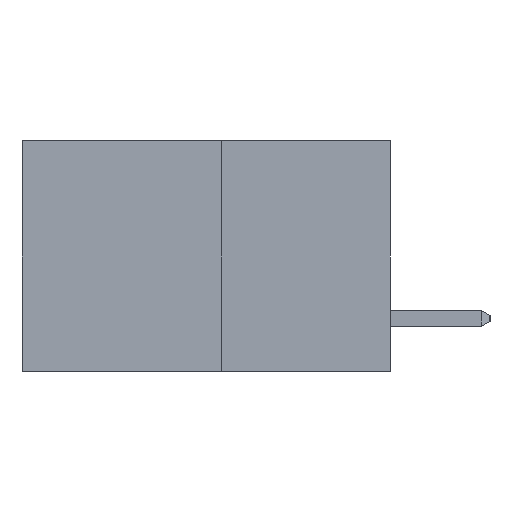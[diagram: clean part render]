
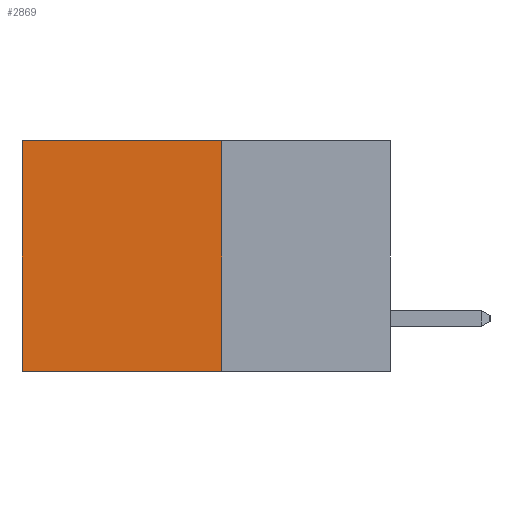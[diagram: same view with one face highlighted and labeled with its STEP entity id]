
A CAD part, left-side view. The second image highlights one B-rep face of the part: STEP entity #2869.
In plain terms, the highlighted planar face has unit normal (-1, 0, 0).
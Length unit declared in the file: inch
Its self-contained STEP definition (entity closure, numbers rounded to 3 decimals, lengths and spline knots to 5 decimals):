
#576 = LINE ( 'NONE', #3985, #7108 ) ;
#730 = DIRECTION ( 'NONE',  ( 0., 1., 0. ) ) ;
#1033 = CARTESIAN_POINT ( 'NONE',  ( 0.277, 0.59, -0.37 ) ) ;
#1286 = DIRECTION ( 'NONE',  ( 0., 0., -1. ) ) ;
#1570 = CARTESIAN_POINT ( 'NONE',  ( 0.277, 0.27, -0.37 ) ) ;
#1592 = LINE ( 'NONE', #6024, #7834 ) ;
#1625 = EDGE_LOOP ( 'NONE', ( #1772, #9178, #2655, #3775 ) ) ;
#1628 = VERTEX_POINT ( 'NONE', #6044 ) ;
#1671 = PLANE ( 'NONE',  #3320 ) ;
#1772 = ORIENTED_EDGE ( 'NONE', *, *, #9728, .T. ) ;
#1929 = VECTOR ( 'NONE', #8327, 39.37008 ) ;
#2655 = ORIENTED_EDGE ( 'NONE', *, *, #8608, .F. ) ;
#2869 = ADVANCED_FACE ( 'NONE', ( #3072 ), #1671, .F. ) ;
#3072 = FACE_OUTER_BOUND ( 'NONE', #1625, .T. ) ;
#3103 = CARTESIAN_POINT ( 'NONE',  ( 0.277, 0.27, 0. ) ) ;
#3320 = AXIS2_PLACEMENT_3D ( 'NONE', #1570, #6896, #9042 ) ;
#3775 = ORIENTED_EDGE ( 'NONE', *, *, #7392, .T. ) ;
#3849 = CARTESIAN_POINT ( 'NONE',  ( 0.277, 0.27, -0.37 ) ) ;
#3985 = CARTESIAN_POINT ( 'NONE',  ( 0.277, 0.27, 0. ) ) ;
#4096 = EDGE_CURVE ( 'NONE', #6271, #1628, #6357, .T. ) ;
#4168 = CARTESIAN_POINT ( 'NONE',  ( 0.277, 0.59, 0. ) ) ;
#4412 = VECTOR ( 'NONE', #9612, 39.37008 ) ;
#5174 = LINE ( 'NONE', #1033, #4412 ) ;
#5218 = VERTEX_POINT ( 'NONE', #4168 ) ;
#6024 = CARTESIAN_POINT ( 'NONE',  ( 0.277, 0.27, -0.37 ) ) ;
#6044 = CARTESIAN_POINT ( 'NONE',  ( 0.277, 0.59, -0.37 ) ) ;
#6271 = VERTEX_POINT ( 'NONE', #6558 ) ;
#6357 = LINE ( 'NONE', #3849, #1929 ) ;
#6558 = CARTESIAN_POINT ( 'NONE',  ( 0.277, 0.27, -0.37 ) ) ;
#6740 = VERTEX_POINT ( 'NONE', #3103 ) ;
#6896 = DIRECTION ( 'NONE',  ( 1., 0., 0. ) ) ;
#7108 = VECTOR ( 'NONE', #730, 39.37008 ) ;
#7392 = EDGE_CURVE ( 'NONE', #6740, #5218, #576, .T. ) ;
#7834 = VECTOR ( 'NONE', #1286, 39.37008 ) ;
#8327 = DIRECTION ( 'NONE',  ( 0., 1., 0. ) ) ;
#8608 = EDGE_CURVE ( 'NONE', #6740, #6271, #1592, .T. ) ;
#9042 = DIRECTION ( 'NONE',  ( 0., 0., -1. ) ) ;
#9178 = ORIENTED_EDGE ( 'NONE', *, *, #4096, .F. ) ;
#9612 = DIRECTION ( 'NONE',  ( 0., 0., -1. ) ) ;
#9728 = EDGE_CURVE ( 'NONE', #5218, #1628, #5174, .T. ) ;
